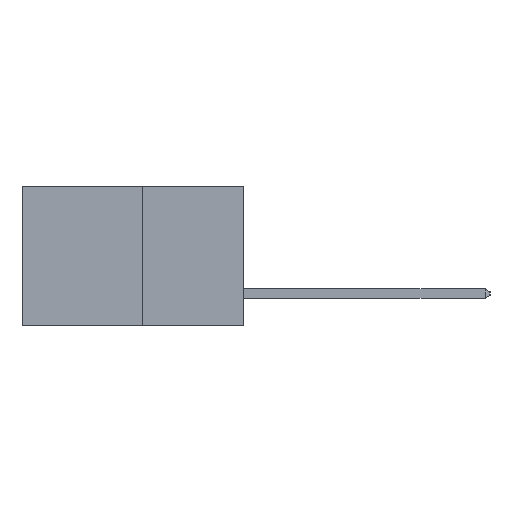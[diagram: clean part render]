
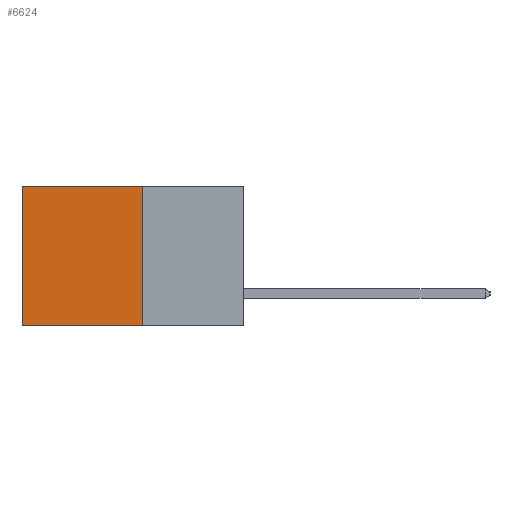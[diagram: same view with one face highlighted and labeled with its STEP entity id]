
A CAD part, left-side view. The second image highlights one B-rep face of the part: STEP entity #6624.
In plain terms, the highlighted planar face has unit normal (-1, 0, 0).
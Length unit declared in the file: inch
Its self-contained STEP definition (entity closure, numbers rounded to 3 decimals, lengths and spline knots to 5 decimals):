
#221 = CARTESIAN_POINT ( 'NONE',  ( 0.277, 0.27, -0.37 ) ) ;
#502 = VECTOR ( 'NONE', #6031, 39.37008 ) ;
#762 = CARTESIAN_POINT ( 'NONE',  ( 0.277, 0.27, 0. ) ) ;
#1177 = CARTESIAN_POINT ( 'NONE',  ( 0.277, 0.27, 0. ) ) ;
#1529 = VERTEX_POINT ( 'NONE', #762 ) ;
#1738 = EDGE_CURVE ( 'NONE', #1529, #6637, #3254, .T. ) ;
#1814 = CARTESIAN_POINT ( 'NONE',  ( 0.277, 0.59, -0.37 ) ) ;
#2953 = VECTOR ( 'NONE', #4940, 39.37008 ) ;
#3254 = LINE ( 'NONE', #1177, #3553 ) ;
#3553 = VECTOR ( 'NONE', #11219, 39.37008 ) ;
#4300 = ORIENTED_EDGE ( 'NONE', *, *, #4403, .F. ) ;
#4403 = EDGE_CURVE ( 'NONE', #5812, #5972, #5975, .T. ) ;
#4602 = ORIENTED_EDGE ( 'NONE', *, *, #4853, .F. ) ;
#4769 = CARTESIAN_POINT ( 'NONE',  ( 0.277, 0.59, -0.37 ) ) ;
#4796 = EDGE_LOOP ( 'NONE', ( #5992, #4300, #4602, #8155 ) ) ;
#4853 = EDGE_CURVE ( 'NONE', #1529, #5812, #10876, .T. ) ;
#4940 = DIRECTION ( 'NONE',  ( 0., 0., -1. ) ) ;
#5197 = CARTESIAN_POINT ( 'NONE',  ( 0.277, 0.27, -0.37 ) ) ;
#5348 = VECTOR ( 'NONE', #8007, 39.37008 ) ;
#5588 = LINE ( 'NONE', #4769, #2953 ) ;
#5812 = VERTEX_POINT ( 'NONE', #5197 ) ;
#5972 = VERTEX_POINT ( 'NONE', #1814 ) ;
#5975 = LINE ( 'NONE', #221, #5348 ) ;
#5992 = ORIENTED_EDGE ( 'NONE', *, *, #6910, .T. ) ;
#6031 = DIRECTION ( 'NONE',  ( 0., 0., -1. ) ) ;
#6600 = CARTESIAN_POINT ( 'NONE',  ( 0.277, 0.27, -0.37 ) ) ;
#6624 = ADVANCED_FACE ( 'NONE', ( #11423 ), #9624, .F. ) ;
#6637 = VERTEX_POINT ( 'NONE', #9317 ) ;
#6910 = EDGE_CURVE ( 'NONE', #6637, #5972, #5588, .T. ) ;
#7005 = AXIS2_PLACEMENT_3D ( 'NONE', #9611, #9536, #9465 ) ;
#8007 = DIRECTION ( 'NONE',  ( 0., 1., 0. ) ) ;
#8155 = ORIENTED_EDGE ( 'NONE', *, *, #1738, .T. ) ;
#9317 = CARTESIAN_POINT ( 'NONE',  ( 0.277, 0.59, 0. ) ) ;
#9465 = DIRECTION ( 'NONE',  ( 0., 0., -1. ) ) ;
#9536 = DIRECTION ( 'NONE',  ( 1., 0., 0. ) ) ;
#9611 = CARTESIAN_POINT ( 'NONE',  ( 0.277, 0.27, -0.37 ) ) ;
#9624 = PLANE ( 'NONE',  #7005 ) ;
#10876 = LINE ( 'NONE', #6600, #502 ) ;
#11219 = DIRECTION ( 'NONE',  ( 0., 1., 0. ) ) ;
#11423 = FACE_OUTER_BOUND ( 'NONE', #4796, .T. ) ;
